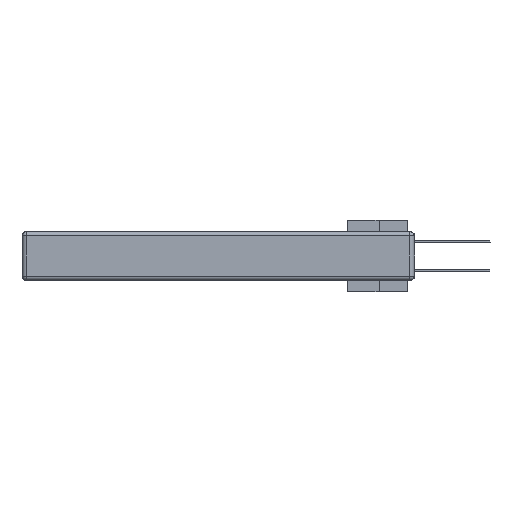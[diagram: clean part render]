
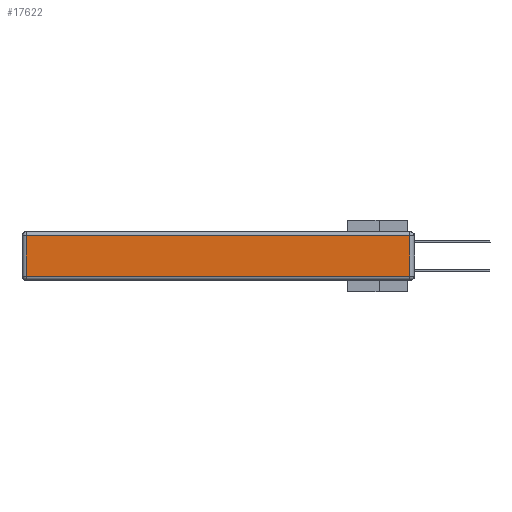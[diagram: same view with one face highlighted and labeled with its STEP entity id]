
A CAD part, left-side view. The second image highlights one B-rep face of the part: STEP entity #17622.
In plain terms, the highlighted planar face has unit normal (-1, 0, 0).
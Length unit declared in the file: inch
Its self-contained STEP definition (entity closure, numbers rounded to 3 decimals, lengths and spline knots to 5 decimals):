
#814 = DIRECTION ( 'NONE',  ( 0., 1., 0. ) ) ;
#1334 = VECTOR ( 'NONE', #3046, 39.37008 ) ;
#1379 = CARTESIAN_POINT ( 'NONE',  ( 0., 0., -0.343 ) ) ;
#1963 = LINE ( 'NONE', #26955, #28797 ) ;
#2872 = VERTEX_POINT ( 'NONE', #20321 ) ;
#3046 = DIRECTION ( 'NONE',  ( 0., 0., -1. ) ) ;
#3107 = CARTESIAN_POINT ( 'NONE',  ( 0., 0., -0.313 ) ) ;
#3659 = PLANE ( 'NONE',  #20955 ) ;
#3905 = CARTESIAN_POINT ( 'NONE',  ( 0., 2.72, -0.03 ) ) ;
#4450 = EDGE_CURVE ( 'NONE', #12133, #12778, #30811, .T. ) ;
#5221 = EDGE_CURVE ( 'NONE', #12778, #2872, #16834, .T. ) ;
#5734 = CARTESIAN_POINT ( 'NONE',  ( 0., 0.03, -0.343 ) ) ;
#6180 = DIRECTION ( 'NONE',  ( 0., 0., 1. ) ) ;
#7216 = ORIENTED_EDGE ( 'NONE', *, *, #4450, .T. ) ;
#7256 = CARTESIAN_POINT ( 'NONE',  ( 0., 0.03, -0.03 ) ) ;
#8688 = VECTOR ( 'NONE', #15033, 39.37008 ) ;
#9494 = CARTESIAN_POINT ( 'NONE',  ( 0., 2.72, -0.343 ) ) ;
#9898 = EDGE_LOOP ( 'NONE', ( #19889, #19662, #14888, #7216 ) ) ;
#11356 = CARTESIAN_POINT ( 'NONE',  ( 0., 2.72, -0.313 ) ) ;
#12133 = VERTEX_POINT ( 'NONE', #3905 ) ;
#12778 = VERTEX_POINT ( 'NONE', #11356 ) ;
#13646 = VERTEX_POINT ( 'NONE', #7256 ) ;
#14888 = ORIENTED_EDGE ( 'NONE', *, *, #20403, .T. ) ;
#15033 = DIRECTION ( 'NONE',  ( 0., -1., 0. ) ) ;
#16834 = LINE ( 'NONE', #3107, #8688 ) ;
#17622 = ADVANCED_FACE ( 'NONE', ( #30501 ), #3659, .T. ) ;
#19662 = ORIENTED_EDGE ( 'NONE', *, *, #27013, .T. ) ;
#19889 = ORIENTED_EDGE ( 'NONE', *, *, #5221, .T. ) ;
#20321 = CARTESIAN_POINT ( 'NONE',  ( 0., 0.03, -0.313 ) ) ;
#20403 = EDGE_CURVE ( 'NONE', #13646, #12133, #1963, .T. ) ;
#20955 = AXIS2_PLACEMENT_3D ( 'NONE', #1379, #27842, #6180 ) ;
#21614 = VECTOR ( 'NONE', #24782, 39.37008 ) ;
#24782 = DIRECTION ( 'NONE',  ( 0., 0., 1. ) ) ;
#26955 = CARTESIAN_POINT ( 'NONE',  ( 0., 2.75, -0.03 ) ) ;
#27013 = EDGE_CURVE ( 'NONE', #2872, #13646, #29108, .T. ) ;
#27842 = DIRECTION ( 'NONE',  ( -1., 0., 0. ) ) ;
#28797 = VECTOR ( 'NONE', #814, 39.37008 ) ;
#29108 = LINE ( 'NONE', #5734, #21614 ) ;
#30501 = FACE_OUTER_BOUND ( 'NONE', #9898, .T. ) ;
#30811 = LINE ( 'NONE', #9494, #1334 ) ;
